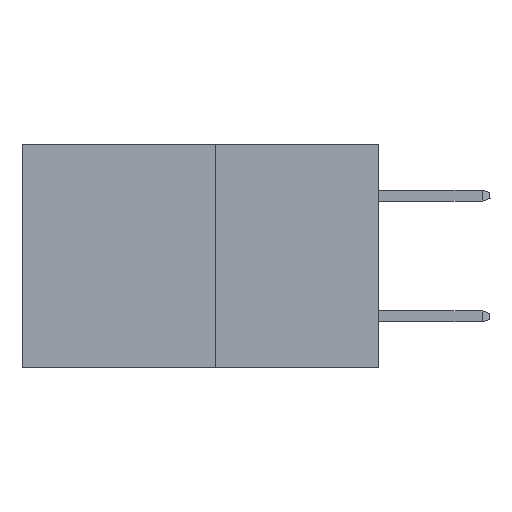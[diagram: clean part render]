
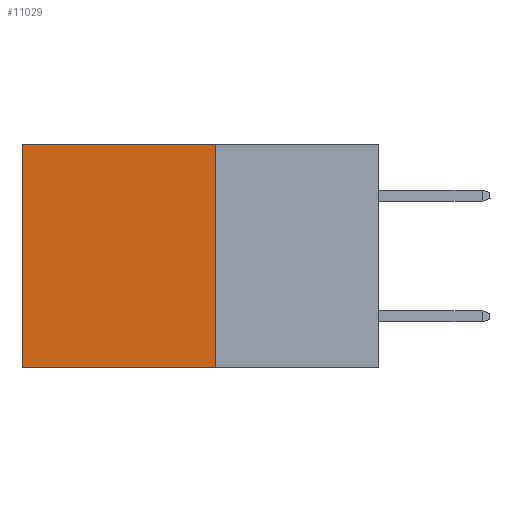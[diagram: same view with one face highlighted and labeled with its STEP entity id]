
A CAD part, left-side view. The second image highlights one B-rep face of the part: STEP entity #11029.
In plain terms, the highlighted planar face has unit normal (-1, 0, 0).
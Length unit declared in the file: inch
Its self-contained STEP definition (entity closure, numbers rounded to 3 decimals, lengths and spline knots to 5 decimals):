
#824 = EDGE_CURVE ( 'NONE', #12443, #9170, #3507, .T. ) ;
#897 = CARTESIAN_POINT ( 'NONE',  ( 0.277, 0.27, -0.37 ) ) ;
#974 = FACE_OUTER_BOUND ( 'NONE', #15250, .T. ) ;
#2742 = DIRECTION ( 'NONE',  ( 0., 1., 0. ) ) ;
#2911 = CARTESIAN_POINT ( 'NONE',  ( 0.277, 0.27, -0.37 ) ) ;
#3507 = LINE ( 'NONE', #19540, #19138 ) ;
#4782 = VERTEX_POINT ( 'NONE', #14517 ) ;
#5107 = CARTESIAN_POINT ( 'NONE',  ( 0.277, 0.59, -0.37 ) ) ;
#5806 = EDGE_CURVE ( 'NONE', #18259, #4782, #10957, .T. ) ;
#6538 = CARTESIAN_POINT ( 'NONE',  ( 0.277, 0.27, -0.37 ) ) ;
#8061 = DIRECTION ( 'NONE',  ( 0., 0., -1. ) ) ;
#8125 = DIRECTION ( 'NONE',  ( 0., 0., -1. ) ) ;
#9170 = VERTEX_POINT ( 'NONE', #17802 ) ;
#9221 = DIRECTION ( 'NONE',  ( 0., 1., 0. ) ) ;
#10606 = EDGE_CURVE ( 'NONE', #12443, #18259, #16787, .T. ) ;
#10725 = AXIS2_PLACEMENT_3D ( 'NONE', #6538, #17553, #8061 ) ;
#10957 = LINE ( 'NONE', #2911, #19306 ) ;
#11029 = ADVANCED_FACE ( 'NONE', ( #974 ), #14439, .F. ) ;
#11498 = ORIENTED_EDGE ( 'NONE', *, *, #14065, .T. ) ;
#11997 = ORIENTED_EDGE ( 'NONE', *, *, #5806, .F. ) ;
#12038 = VECTOR ( 'NONE', #15153, 39.37008 ) ;
#12443 = VERTEX_POINT ( 'NONE', #20008 ) ;
#14065 = EDGE_CURVE ( 'NONE', #9170, #4782, #18249, .T. ) ;
#14170 = VECTOR ( 'NONE', #8125, 39.37008 ) ;
#14346 = ORIENTED_EDGE ( 'NONE', *, *, #824, .T. ) ;
#14439 = PLANE ( 'NONE',  #10725 ) ;
#14517 = CARTESIAN_POINT ( 'NONE',  ( 0.277, 0.59, -0.37 ) ) ;
#14622 = CARTESIAN_POINT ( 'NONE',  ( 0.277, 0.27, -0.37 ) ) ;
#15153 = DIRECTION ( 'NONE',  ( 0., 0., -1. ) ) ;
#15250 = EDGE_LOOP ( 'NONE', ( #11498, #11997, #16579, #14346 ) ) ;
#16579 = ORIENTED_EDGE ( 'NONE', *, *, #10606, .F. ) ;
#16787 = LINE ( 'NONE', #897, #12038 ) ;
#17553 = DIRECTION ( 'NONE',  ( 1., 0., 0. ) ) ;
#17802 = CARTESIAN_POINT ( 'NONE',  ( 0.277, 0.59, 0. ) ) ;
#18249 = LINE ( 'NONE', #5107, #14170 ) ;
#18259 = VERTEX_POINT ( 'NONE', #14622 ) ;
#19138 = VECTOR ( 'NONE', #9221, 39.37008 ) ;
#19306 = VECTOR ( 'NONE', #2742, 39.37008 ) ;
#19540 = CARTESIAN_POINT ( 'NONE',  ( 0.277, 0.27, 0. ) ) ;
#20008 = CARTESIAN_POINT ( 'NONE',  ( 0.277, 0.27, 0. ) ) ;
